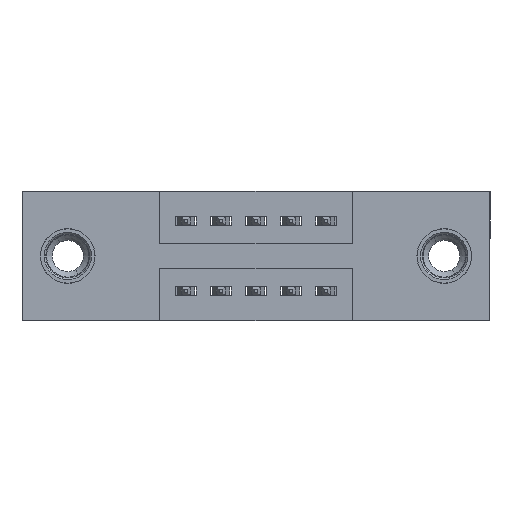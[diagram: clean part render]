
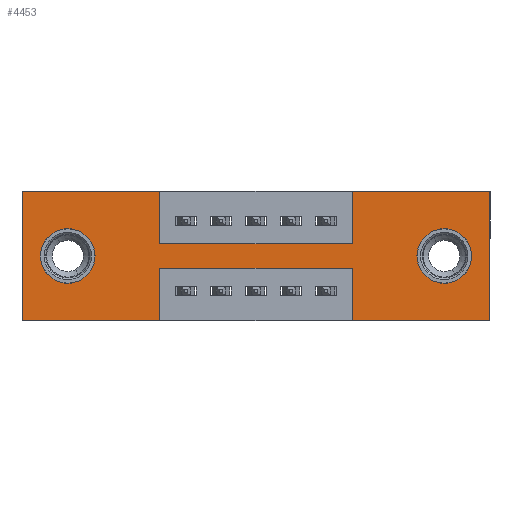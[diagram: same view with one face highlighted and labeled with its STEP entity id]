
A CAD part, front view. The second image highlights one B-rep face of the part: STEP entity #4453.
In plain terms, the highlighted planar face has unit normal (0, -1, 0).
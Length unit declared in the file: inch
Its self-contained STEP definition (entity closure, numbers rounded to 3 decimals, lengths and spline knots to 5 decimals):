
#110 = VERTEX_POINT ( 'NONE', #7260 ) ;
#331 = AXIS2_PLACEMENT_3D ( 'NONE', #4159, #10111, #5060 ) ;
#412 = VERTEX_POINT ( 'NONE', #10578 ) ;
#498 = CARTESIAN_POINT ( 'NONE',  ( 0.3925, 0., -0.22 ) ) ;
#515 = EDGE_LOOP ( 'NONE', ( #2851, #5423 ) ) ;
#615 = CARTESIAN_POINT ( 'NONE',  ( 0.3925, 0., 0. ) ) ;
#665 = VECTOR ( 'NONE', #2413, 39.37008 ) ;
#706 = VERTEX_POINT ( 'NONE', #825 ) ;
#825 = CARTESIAN_POINT ( 'NONE',  ( 0.3925, 0., -0.22 ) ) ;
#981 = ORIENTED_EDGE ( 'NONE', *, *, #7442, .T. ) ;
#989 = CARTESIAN_POINT ( 'NONE',  ( 0., 0., -0.37 ) ) ;
#1063 = LINE ( 'NONE', #5825, #9908 ) ;
#1075 = CARTESIAN_POINT ( 'NONE',  ( 1.335, 0., 0. ) ) ;
#1239 = FACE_OUTER_BOUND ( 'NONE', #1741, .T. ) ;
#1482 = VECTOR ( 'NONE', #7525, 39.37008 ) ;
#1539 = VERTEX_POINT ( 'NONE', #10067 ) ;
#1563 = DIRECTION ( 'NONE',  ( 0., -1., 0. ) ) ;
#1671 = VECTOR ( 'NONE', #10753, 39.37008 ) ;
#1699 = CARTESIAN_POINT ( 'NONE',  ( 0., 0., 0. ) ) ;
#1741 = EDGE_LOOP ( 'NONE', ( #6844, #9574, #2131, #2685, #8292, #9124, #2562, #8655, #7708, #6113, #9322, #4599 ) ) ;
#1754 = EDGE_CURVE ( 'NONE', #8059, #2197, #2238, .T. ) ;
#1996 = LINE ( 'NONE', #3367, #10781 ) ;
#2051 = CIRCLE ( 'NONE', #9412, 0.078 ) ;
#2092 = EDGE_LOOP ( 'NONE', ( #2290, #981 ) ) ;
#2131 = ORIENTED_EDGE ( 'NONE', *, *, #6482, .F. ) ;
#2197 = VERTEX_POINT ( 'NONE', #7031 ) ;
#2238 = LINE ( 'NONE', #1699, #11008 ) ;
#2290 = ORIENTED_EDGE ( 'NONE', *, *, #4377, .T. ) ;
#2336 = CARTESIAN_POINT ( 'NONE',  ( 0., 0., -0.37 ) ) ;
#2413 = DIRECTION ( 'NONE',  ( 0., 0., 1. ) ) ;
#2448 = AXIS2_PLACEMENT_3D ( 'NONE', #6468, #1563, #4297 ) ;
#2562 = ORIENTED_EDGE ( 'NONE', *, *, #8646, .F. ) ;
#2672 = EDGE_CURVE ( 'NONE', #10219, #110, #7912, .T. ) ;
#2685 = ORIENTED_EDGE ( 'NONE', *, *, #7909, .F. ) ;
#2836 = LINE ( 'NONE', #3887, #9400 ) ;
#2847 = LINE ( 'NONE', #1075, #8896 ) ;
#2851 = ORIENTED_EDGE ( 'NONE', *, *, #2672, .T. ) ;
#3000 = CARTESIAN_POINT ( 'NONE',  ( 0.9425, 0., -0.15 ) ) ;
#3080 = CARTESIAN_POINT ( 'NONE',  ( 0., 0., -0.37 ) ) ;
#3233 = DIRECTION ( 'NONE',  ( 1., 0., 0. ) ) ;
#3367 = CARTESIAN_POINT ( 'NONE',  ( 0.3925, 0., -0.15 ) ) ;
#3444 = EDGE_CURVE ( 'NONE', #4865, #8967, #6963, .T. ) ;
#3540 = FACE_BOUND ( 'NONE', #515, .T. ) ;
#3694 = CARTESIAN_POINT ( 'NONE',  ( 0.9425, 0., -0.37 ) ) ;
#3887 = CARTESIAN_POINT ( 'NONE',  ( 0., 0., 0. ) ) ;
#3983 = DIRECTION ( 'NONE',  ( -1., 0., 0. ) ) ;
#4017 = CARTESIAN_POINT ( 'NONE',  ( 0.3925, 0., 0. ) ) ;
#4038 = LINE ( 'NONE', #2336, #1482 ) ;
#4159 = CARTESIAN_POINT ( 'NONE',  ( 1.205, 0., -0.185 ) ) ;
#4297 = DIRECTION ( 'NONE',  ( 0., 0., -1. ) ) ;
#4301 = DIRECTION ( 'NONE',  ( 0., 0., -1. ) ) ;
#4377 = EDGE_CURVE ( 'NONE', #10685, #7813, #2051, .T. ) ;
#4453 = ADVANCED_FACE ( 'NONE', ( #6401, #3540, #1239 ), #5602, .T. ) ;
#4504 = VERTEX_POINT ( 'NONE', #989 ) ;
#4599 = ORIENTED_EDGE ( 'NONE', *, *, #10296, .F. ) ;
#4854 = CARTESIAN_POINT ( 'NONE',  ( 0.13, 0., -0.107 ) ) ;
#4865 = VERTEX_POINT ( 'NONE', #4017 ) ;
#4927 = CARTESIAN_POINT ( 'NONE',  ( 0.13, 0., -0.185 ) ) ;
#5060 = DIRECTION ( 'NONE',  ( 0., 0., -1. ) ) ;
#5097 = DIRECTION ( 'NONE',  ( 0., 1., 0. ) ) ;
#5146 = DIRECTION ( 'NONE',  ( 0., 1., 0. ) ) ;
#5240 = LINE ( 'NONE', #10433, #9476 ) ;
#5358 = VERTEX_POINT ( 'NONE', #3000 ) ;
#5423 = ORIENTED_EDGE ( 'NONE', *, *, #8074, .T. ) ;
#5461 = CARTESIAN_POINT ( 'NONE',  ( 0.3925, 0., -0.15 ) ) ;
#5481 = VERTEX_POINT ( 'NONE', #8311 ) ;
#5504 = VERTEX_POINT ( 'NONE', #10044 ) ;
#5577 = DIRECTION ( 'NONE',  ( 0., 0., 1. ) ) ;
#5602 = PLANE ( 'NONE',  #2448 ) ;
#5703 = CARTESIAN_POINT ( 'NONE',  ( 0.3925, 0., -0.37 ) ) ;
#5825 = CARTESIAN_POINT ( 'NONE',  ( 0., 0., 0. ) ) ;
#6028 = VECTOR ( 'NONE', #3983, 39.37008 ) ;
#6113 = ORIENTED_EDGE ( 'NONE', *, *, #6738, .F. ) ;
#6290 = LINE ( 'NONE', #498, #6028 ) ;
#6368 = VECTOR ( 'NONE', #7997, 39.37008 ) ;
#6401 = FACE_BOUND ( 'NONE', #2092, .T. ) ;
#6456 = CARTESIAN_POINT ( 'NONE',  ( 1.205, 0., -0.263 ) ) ;
#6464 = EDGE_CURVE ( 'NONE', #2197, #5481, #2847, .T. ) ;
#6468 = CARTESIAN_POINT ( 'NONE',  ( 0., 0., -0.37 ) ) ;
#6482 = EDGE_CURVE ( 'NONE', #412, #5504, #8634, .T. ) ;
#6526 = DIRECTION ( 'NONE',  ( 0., 0., 1. ) ) ;
#6738 = EDGE_CURVE ( 'NONE', #1539, #4865, #1063, .T. ) ;
#6741 = CARTESIAN_POINT ( 'NONE',  ( 0.9425, 0., 0. ) ) ;
#6844 = ORIENTED_EDGE ( 'NONE', *, *, #7146, .F. ) ;
#6953 = CIRCLE ( 'NONE', #10486, 0.078 ) ;
#6963 = LINE ( 'NONE', #615, #8944 ) ;
#7031 = CARTESIAN_POINT ( 'NONE',  ( 1.335, 0., 0. ) ) ;
#7146 = EDGE_CURVE ( 'NONE', #706, #7889, #5240, .T. ) ;
#7233 = DIRECTION ( 'NONE',  ( 0., 1., 0. ) ) ;
#7260 = CARTESIAN_POINT ( 'NONE',  ( 0.13, 0., -0.263 ) ) ;
#7442 = EDGE_CURVE ( 'NONE', #7813, #10685, #10727, .T. ) ;
#7525 = DIRECTION ( 'NONE',  ( -1., 0., 0. ) ) ;
#7705 = CARTESIAN_POINT ( 'NONE',  ( 1.205, 0., -0.185 ) ) ;
#7708 = ORIENTED_EDGE ( 'NONE', *, *, #3444, .F. ) ;
#7813 = VERTEX_POINT ( 'NONE', #6456 ) ;
#7889 = VERTEX_POINT ( 'NONE', #5703 ) ;
#7909 = EDGE_CURVE ( 'NONE', #5481, #412, #8820, .T. ) ;
#7912 = CIRCLE ( 'NONE', #9334, 0.078 ) ;
#7938 = EDGE_CURVE ( 'NONE', #5504, #706, #6290, .T. ) ;
#7997 = DIRECTION ( 'NONE',  ( 0., 0., 1. ) ) ;
#8059 = VERTEX_POINT ( 'NONE', #8501 ) ;
#8074 = EDGE_CURVE ( 'NONE', #110, #10219, #6953, .T. ) ;
#8292 = ORIENTED_EDGE ( 'NONE', *, *, #6464, .F. ) ;
#8311 = CARTESIAN_POINT ( 'NONE',  ( 1.335, 0., -0.37 ) ) ;
#8336 = DIRECTION ( 'NONE',  ( 1., 0., 0. ) ) ;
#8501 = CARTESIAN_POINT ( 'NONE',  ( 0.9425, 0., 0. ) ) ;
#8530 = DIRECTION ( 'NONE',  ( 1., 0., 0. ) ) ;
#8634 = LINE ( 'NONE', #3694, #6368 ) ;
#8646 = EDGE_CURVE ( 'NONE', #5358, #8059, #9812, .T. ) ;
#8655 = ORIENTED_EDGE ( 'NONE', *, *, #10705, .F. ) ;
#8815 = DIRECTION ( 'NONE',  ( 0., 0., -1. ) ) ;
#8820 = LINE ( 'NONE', #3080, #1671 ) ;
#8896 = VECTOR ( 'NONE', #8815, 39.37008 ) ;
#8944 = VECTOR ( 'NONE', #10766, 39.37008 ) ;
#8967 = VERTEX_POINT ( 'NONE', #5461 ) ;
#9124 = ORIENTED_EDGE ( 'NONE', *, *, #1754, .F. ) ;
#9322 = ORIENTED_EDGE ( 'NONE', *, *, #10172, .F. ) ;
#9334 = AXIS2_PLACEMENT_3D ( 'NONE', #4927, #5097, #5577 ) ;
#9400 = VECTOR ( 'NONE', #6526, 39.37008 ) ;
#9412 = AXIS2_PLACEMENT_3D ( 'NONE', #7705, #7233, #4301 ) ;
#9476 = VECTOR ( 'NONE', #9689, 39.37008 ) ;
#9574 = ORIENTED_EDGE ( 'NONE', *, *, #7938, .F. ) ;
#9689 = DIRECTION ( 'NONE',  ( 0., 0., -1. ) ) ;
#9812 = LINE ( 'NONE', #6741, #665 ) ;
#9908 = VECTOR ( 'NONE', #3233, 39.37008 ) ;
#10044 = CARTESIAN_POINT ( 'NONE',  ( 0.9425, 0., -0.22 ) ) ;
#10067 = CARTESIAN_POINT ( 'NONE',  ( 0., 0., 0. ) ) ;
#10111 = DIRECTION ( 'NONE',  ( 0., 1., 0. ) ) ;
#10145 = CARTESIAN_POINT ( 'NONE',  ( 1.205, 0., -0.107 ) ) ;
#10172 = EDGE_CURVE ( 'NONE', #4504, #1539, #2836, .T. ) ;
#10187 = CARTESIAN_POINT ( 'NONE',  ( 0.13, 0., -0.185 ) ) ;
#10219 = VERTEX_POINT ( 'NONE', #4854 ) ;
#10296 = EDGE_CURVE ( 'NONE', #7889, #4504, #4038, .T. ) ;
#10433 = CARTESIAN_POINT ( 'NONE',  ( 0.3925, 0., -0.37 ) ) ;
#10486 = AXIS2_PLACEMENT_3D ( 'NONE', #10187, #5146, #10993 ) ;
#10578 = CARTESIAN_POINT ( 'NONE',  ( 0.9425, 0., -0.37 ) ) ;
#10685 = VERTEX_POINT ( 'NONE', #10145 ) ;
#10705 = EDGE_CURVE ( 'NONE', #8967, #5358, #1996, .T. ) ;
#10727 = CIRCLE ( 'NONE', #331, 0.078 ) ;
#10753 = DIRECTION ( 'NONE',  ( -1., 0., 0. ) ) ;
#10766 = DIRECTION ( 'NONE',  ( 0., 0., -1. ) ) ;
#10781 = VECTOR ( 'NONE', #8530, 39.37008 ) ;
#10993 = DIRECTION ( 'NONE',  ( 0., 0., 1. ) ) ;
#11008 = VECTOR ( 'NONE', #8336, 39.37008 ) ;
